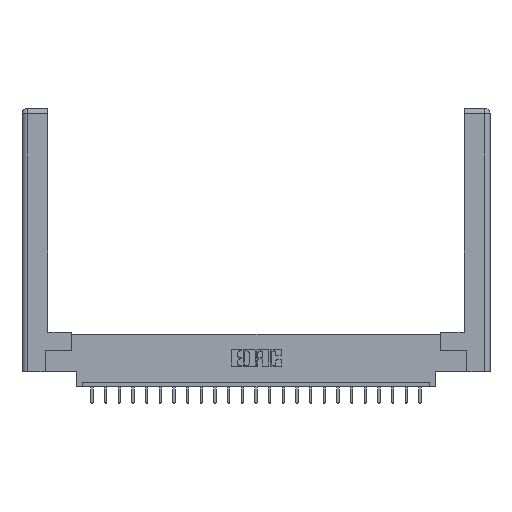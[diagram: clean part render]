
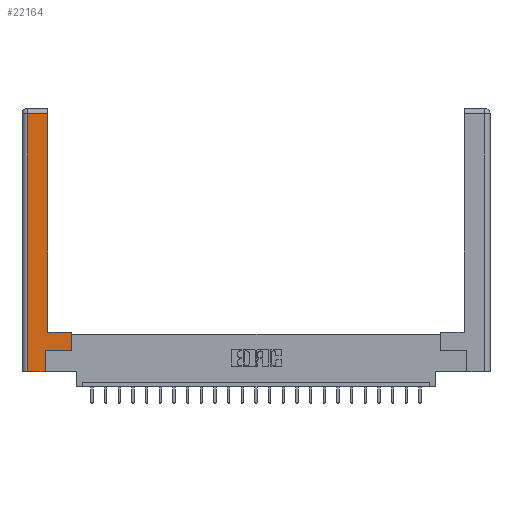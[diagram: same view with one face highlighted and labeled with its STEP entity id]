
A CAD part, top view. The second image highlights one B-rep face of the part: STEP entity #22164.
In plain terms, the highlighted planar face has unit normal (0, 0, 1).
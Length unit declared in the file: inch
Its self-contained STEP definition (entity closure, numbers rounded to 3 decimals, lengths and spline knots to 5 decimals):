
#903 = FACE_OUTER_BOUND ( 'NONE', #5816, .T. ) ;
#1024 = DIRECTION ( 'NONE',  ( -1., 0., 0. ) ) ;
#1031 = DIRECTION ( 'NONE',  ( 0., 0., -1. ) ) ;
#1337 = CARTESIAN_POINT ( 'NONE',  ( 0.565, 0.45, 0. ) ) ;
#1367 = CARTESIAN_POINT ( 'NONE',  ( 0.0615, 0., 0. ) ) ;
#1527 = AXIS2_PLACEMENT_3D ( 'NONE', #15307, #1031, #10079 ) ;
#1981 = VERTEX_POINT ( 'NONE', #23215 ) ;
#2116 = ORIENTED_EDGE ( 'NONE', *, *, #22279, .T. ) ;
#2689 = CARTESIAN_POINT ( 'NONE',  ( 0.265, 0.245, 0. ) ) ;
#2828 = LINE ( 'NONE', #14040, #11398 ) ;
#3304 = LINE ( 'NONE', #1367, #11000 ) ;
#3505 = VECTOR ( 'NONE', #4728, 39.37008 ) ;
#4083 = LINE ( 'NONE', #15620, #3505 ) ;
#4370 = VERTEX_POINT ( 'NONE', #12239 ) ;
#4728 = DIRECTION ( 'NONE',  ( -1., 0., 0. ) ) ;
#5496 = VECTOR ( 'NONE', #20546, 39.37008 ) ;
#5816 = EDGE_LOOP ( 'NONE', ( #18276, #17197, #23053, #20650, #2116, #21005, #12009, #10204 ) ) ;
#6419 = PLANE ( 'NONE',  #1527 ) ;
#7773 = CARTESIAN_POINT ( 'NONE',  ( 0.0615, 0., 0. ) ) ;
#8337 = VECTOR ( 'NONE', #8558, 39.37008 ) ;
#8439 = CARTESIAN_POINT ( 'NONE',  ( 0.0615, 2.94, 0. ) ) ;
#8558 = DIRECTION ( 'NONE',  ( 0., 1., 0. ) ) ;
#8650 = VERTEX_POINT ( 'NONE', #8439 ) ;
#8797 = EDGE_CURVE ( 'NONE', #8650, #14420, #3304, .T. ) ;
#8903 = DIRECTION ( 'NONE',  ( 0., -1., 0. ) ) ;
#8988 = VERTEX_POINT ( 'NONE', #21722 ) ;
#9181 = LINE ( 'NONE', #15839, #8337 ) ;
#9262 = EDGE_CURVE ( 'NONE', #4370, #19864, #10422, .T. ) ;
#10079 = DIRECTION ( 'NONE',  ( -1., 0., 0. ) ) ;
#10135 = EDGE_CURVE ( 'NONE', #13516, #8650, #13184, .T. ) ;
#10204 = ORIENTED_EDGE ( 'NONE', *, *, #18346, .T. ) ;
#10381 = DIRECTION ( 'NONE',  ( 0., 1., 0. ) ) ;
#10422 = LINE ( 'NONE', #1337, #22970 ) ;
#10928 = VECTOR ( 'NONE', #1024, 39.37008 ) ;
#11000 = VECTOR ( 'NONE', #8903, 39.37008 ) ;
#11398 = VECTOR ( 'NONE', #19224, 39.37008 ) ;
#12009 = ORIENTED_EDGE ( 'NONE', *, *, #9262, .T. ) ;
#12239 = CARTESIAN_POINT ( 'NONE',  ( 0.565, 0.245, 0. ) ) ;
#12463 = CARTESIAN_POINT ( 'NONE',  ( 0.295, 3., 0. ) ) ;
#12741 = VERTEX_POINT ( 'NONE', #2689 ) ;
#12930 = EDGE_CURVE ( 'NONE', #14420, #1981, #2828, .T. ) ;
#12960 = CARTESIAN_POINT ( 'NONE',  ( 0.565, 0.245, 0. ) ) ;
#13184 = LINE ( 'NONE', #15682, #10928 ) ;
#13516 = VERTEX_POINT ( 'NONE', #23062 ) ;
#14040 = CARTESIAN_POINT ( 'NONE',  ( 0.265, 0., 0. ) ) ;
#14420 = VERTEX_POINT ( 'NONE', #7773 ) ;
#15307 = CARTESIAN_POINT ( 'NONE',  ( 0., 0., 0. ) ) ;
#15620 = CARTESIAN_POINT ( 'NONE',  ( 0.295, 0.45, 0. ) ) ;
#15682 = CARTESIAN_POINT ( 'NONE',  ( 0.0615, 2.94, 0. ) ) ;
#15839 = CARTESIAN_POINT ( 'NONE',  ( 0.265, 0.245, 0. ) ) ;
#15896 = EDGE_CURVE ( 'NONE', #8988, #13516, #19580, .T. ) ;
#17197 = ORIENTED_EDGE ( 'NONE', *, *, #10135, .T. ) ;
#17920 = DIRECTION ( 'NONE',  ( 0., 1., 0. ) ) ;
#18276 = ORIENTED_EDGE ( 'NONE', *, *, #15896, .T. ) ;
#18346 = EDGE_CURVE ( 'NONE', #19864, #8988, #4083, .T. ) ;
#18434 = VECTOR ( 'NONE', #17920, 39.37008 ) ;
#18612 = LINE ( 'NONE', #12960, #5496 ) ;
#19224 = DIRECTION ( 'NONE',  ( 1., 0., 0. ) ) ;
#19580 = LINE ( 'NONE', #12463, #18434 ) ;
#19864 = VERTEX_POINT ( 'NONE', #21738 ) ;
#20546 = DIRECTION ( 'NONE',  ( 1., 0., 0. ) ) ;
#20650 = ORIENTED_EDGE ( 'NONE', *, *, #12930, .T. ) ;
#21005 = ORIENTED_EDGE ( 'NONE', *, *, #21350, .T. ) ;
#21350 = EDGE_CURVE ( 'NONE', #12741, #4370, #18612, .T. ) ;
#21722 = CARTESIAN_POINT ( 'NONE',  ( 0.295, 0.45, 0. ) ) ;
#21738 = CARTESIAN_POINT ( 'NONE',  ( 0.565, 0.45, 0. ) ) ;
#22164 = ADVANCED_FACE ( 'NONE', ( #903 ), #6419, .F. ) ;
#22279 = EDGE_CURVE ( 'NONE', #1981, #12741, #9181, .T. ) ;
#22970 = VECTOR ( 'NONE', #10381, 39.37008 ) ;
#23053 = ORIENTED_EDGE ( 'NONE', *, *, #8797, .T. ) ;
#23062 = CARTESIAN_POINT ( 'NONE',  ( 0.295, 2.94, 0. ) ) ;
#23215 = CARTESIAN_POINT ( 'NONE',  ( 0.265, 0., 0. ) ) ;
